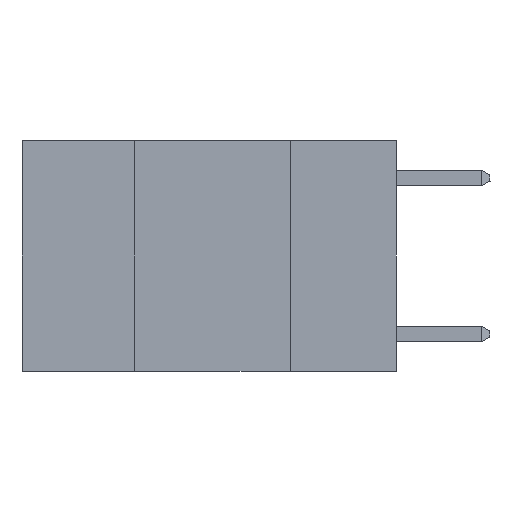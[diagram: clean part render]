
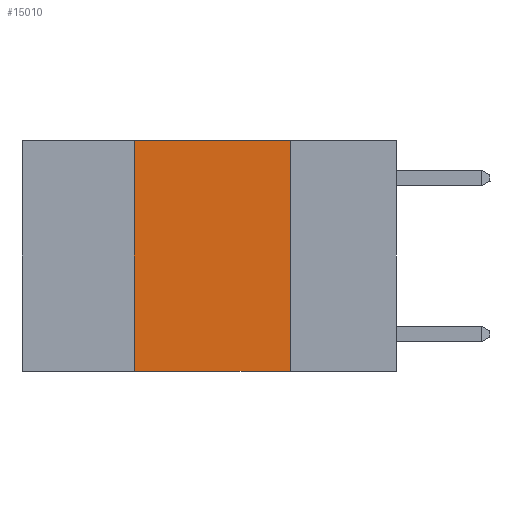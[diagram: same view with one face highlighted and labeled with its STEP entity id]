
A CAD part, left-side view. The second image highlights one B-rep face of the part: STEP entity #15010.
In plain terms, the highlighted planar face has unit normal (-1, 0, 0).
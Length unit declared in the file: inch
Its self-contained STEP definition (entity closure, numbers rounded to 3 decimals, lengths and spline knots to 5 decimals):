
#505 = EDGE_CURVE ( 'NONE', #16375, #27459, #26473, .T. ) ;
#1201 = CARTESIAN_POINT ( 'NONE',  ( 0., 0.42, 0. ) ) ;
#1992 = DIRECTION ( 'NONE',  ( 0., 0., -1. ) ) ;
#2550 = VERTEX_POINT ( 'NONE', #3588 ) ;
#3141 = LINE ( 'NONE', #11182, #25993 ) ;
#3517 = EDGE_CURVE ( 'NONE', #16375, #10227, #3141, .T. ) ;
#3588 = CARTESIAN_POINT ( 'NONE',  ( 0., 0.17, 0. ) ) ;
#4584 = DIRECTION ( 'NONE',  ( 0., -1., 0. ) ) ;
#4893 = AXIS2_PLACEMENT_3D ( 'NONE', #28470, #15281, #1992 ) ;
#4926 = DIRECTION ( 'NONE',  ( 0., 0., -1. ) ) ;
#5681 = VECTOR ( 'NONE', #4926, 39.37008 ) ;
#5819 = ORIENTED_EDGE ( 'NONE', *, *, #26214, .F. ) ;
#7316 = CARTESIAN_POINT ( 'NONE',  ( 0., 0.17, -0.37 ) ) ;
#8884 = VECTOR ( 'NONE', #18815, 39.37008 ) ;
#10227 = VERTEX_POINT ( 'NONE', #7316 ) ;
#10677 = DIRECTION ( 'NONE',  ( 0., -1., 0. ) ) ;
#11182 = CARTESIAN_POINT ( 'NONE',  ( 0., 0.6, -0.37 ) ) ;
#12002 = LINE ( 'NONE', #15059, #28175 ) ;
#13078 = PLANE ( 'NONE',  #4893 ) ;
#14342 = CARTESIAN_POINT ( 'NONE',  ( 0., 0.42, 0. ) ) ;
#14833 = ORIENTED_EDGE ( 'NONE', *, *, #27769, .F. ) ;
#15010 = ADVANCED_FACE ( 'NONE', ( #17676 ), #13078, .F. ) ;
#15059 = CARTESIAN_POINT ( 'NONE',  ( 0., 0.6, 0. ) ) ;
#15281 = DIRECTION ( 'NONE',  ( 1., 0., 0. ) ) ;
#15497 = ORIENTED_EDGE ( 'NONE', *, *, #505, .F. ) ;
#16150 = EDGE_LOOP ( 'NONE', ( #14833, #5819, #15497, #23804 ) ) ;
#16375 = VERTEX_POINT ( 'NONE', #26964 ) ;
#17676 = FACE_OUTER_BOUND ( 'NONE', #16150, .T. ) ;
#18815 = DIRECTION ( 'NONE',  ( 0., 0., 1. ) ) ;
#20328 = CARTESIAN_POINT ( 'NONE',  ( 0., 0.17, 0. ) ) ;
#23804 = ORIENTED_EDGE ( 'NONE', *, *, #3517, .T. ) ;
#24706 = LINE ( 'NONE', #20328, #5681 ) ;
#25993 = VECTOR ( 'NONE', #4584, 39.37008 ) ;
#26214 = EDGE_CURVE ( 'NONE', #27459, #2550, #12002, .T. ) ;
#26473 = LINE ( 'NONE', #14342, #8884 ) ;
#26964 = CARTESIAN_POINT ( 'NONE',  ( 0., 0.42, -0.37 ) ) ;
#27459 = VERTEX_POINT ( 'NONE', #1201 ) ;
#27769 = EDGE_CURVE ( 'NONE', #2550, #10227, #24706, .T. ) ;
#28175 = VECTOR ( 'NONE', #10677, 39.37008 ) ;
#28470 = CARTESIAN_POINT ( 'NONE',  ( 0., 0.6, 0. ) ) ;
